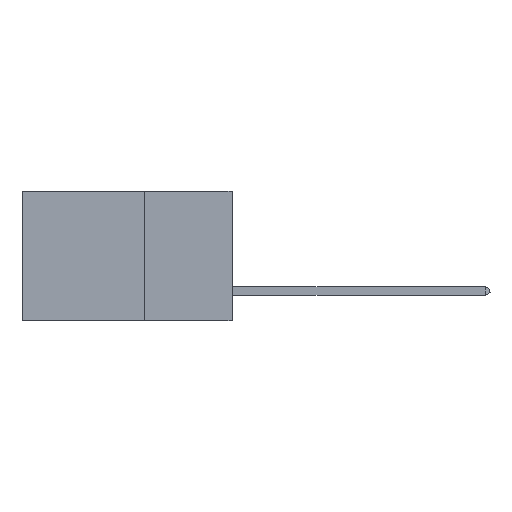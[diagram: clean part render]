
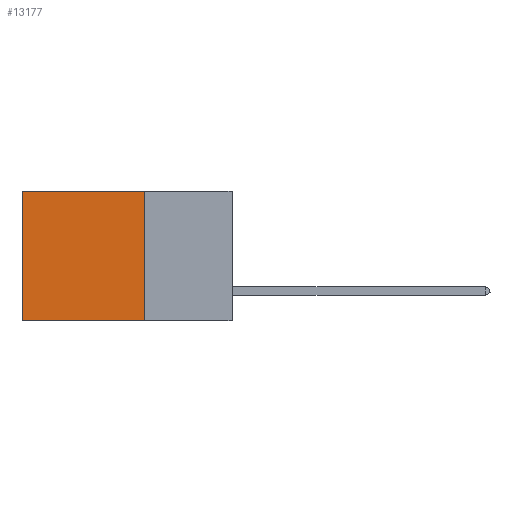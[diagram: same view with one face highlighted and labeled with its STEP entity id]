
A CAD part, left-side view. The second image highlights one B-rep face of the part: STEP entity #13177.
In plain terms, the highlighted planar face has unit normal (-1, 0, 0).
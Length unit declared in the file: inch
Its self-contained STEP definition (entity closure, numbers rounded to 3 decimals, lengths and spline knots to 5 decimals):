
#76 = ORIENTED_EDGE ( 'NONE', *, *, #15622, .F. ) ;
#464 = CARTESIAN_POINT ( 'NONE',  ( 0.2875, 0.6, 0. ) ) ;
#3298 = VERTEX_POINT ( 'NONE', #464 ) ;
#4100 = VERTEX_POINT ( 'NONE', #23570 ) ;
#4575 = CARTESIAN_POINT ( 'NONE',  ( 0.2875, 0.25, 0. ) ) ;
#5204 = LINE ( 'NONE', #13262, #14588 ) ;
#5329 = DIRECTION ( 'NONE',  ( 0., 1., 0. ) ) ;
#6183 = ORIENTED_EDGE ( 'NONE', *, *, #18226, .F. ) ;
#6632 = ORIENTED_EDGE ( 'NONE', *, *, #11803, .T. ) ;
#7379 = VERTEX_POINT ( 'NONE', #4575 ) ;
#8483 = EDGE_CURVE ( 'NONE', #3298, #4100, #5204, .T. ) ;
#8518 = PLANE ( 'NONE',  #15782 ) ;
#9865 = CARTESIAN_POINT ( 'NONE',  ( 0.2875, 0.25, 0. ) ) ;
#9884 = FACE_OUTER_BOUND ( 'NONE', #21790, .T. ) ;
#10629 = VECTOR ( 'NONE', #5329, 39.37008 ) ;
#11803 = EDGE_CURVE ( 'NONE', #7379, #3298, #16961, .T. ) ;
#12140 = LINE ( 'NONE', #17909, #16816 ) ;
#12653 = ORIENTED_EDGE ( 'NONE', *, *, #8483, .T. ) ;
#13177 = ADVANCED_FACE ( 'NONE', ( #9884 ), #8518, .F. ) ;
#13262 = CARTESIAN_POINT ( 'NONE',  ( 0.2875, 0.6, 0. ) ) ;
#14434 = DIRECTION ( 'NONE',  ( 0., 0., -1. ) ) ;
#14588 = VECTOR ( 'NONE', #17140, 39.37008 ) ;
#15609 = DIRECTION ( 'NONE',  ( 0., 1., 0. ) ) ;
#15622 = EDGE_CURVE ( 'NONE', #20557, #4100, #20558, .T. ) ;
#15782 = AXIS2_PLACEMENT_3D ( 'NONE', #23608, #21907, #14434 ) ;
#16816 = VECTOR ( 'NONE', #17316, 39.37008 ) ;
#16823 = CARTESIAN_POINT ( 'NONE',  ( 0.2875, 0.25, -0.37 ) ) ;
#16961 = LINE ( 'NONE', #9865, #20167 ) ;
#17140 = DIRECTION ( 'NONE',  ( 0., 0., -1. ) ) ;
#17240 = CARTESIAN_POINT ( 'NONE',  ( 0.2875, 0.25, -0.37 ) ) ;
#17316 = DIRECTION ( 'NONE',  ( 0., 0., -1. ) ) ;
#17909 = CARTESIAN_POINT ( 'NONE',  ( 0.2875, 0.25, 0. ) ) ;
#18226 = EDGE_CURVE ( 'NONE', #7379, #20557, #12140, .T. ) ;
#20167 = VECTOR ( 'NONE', #15609, 39.37008 ) ;
#20557 = VERTEX_POINT ( 'NONE', #16823 ) ;
#20558 = LINE ( 'NONE', #17240, #10629 ) ;
#21790 = EDGE_LOOP ( 'NONE', ( #12653, #76, #6183, #6632 ) ) ;
#21907 = DIRECTION ( 'NONE',  ( 1., 0., 0. ) ) ;
#23570 = CARTESIAN_POINT ( 'NONE',  ( 0.2875, 0.6, -0.37 ) ) ;
#23608 = CARTESIAN_POINT ( 'NONE',  ( 0.2875, 0.25, 0. ) ) ;
